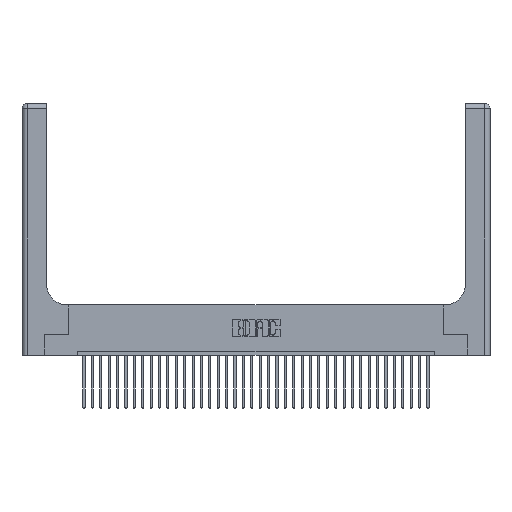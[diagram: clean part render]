
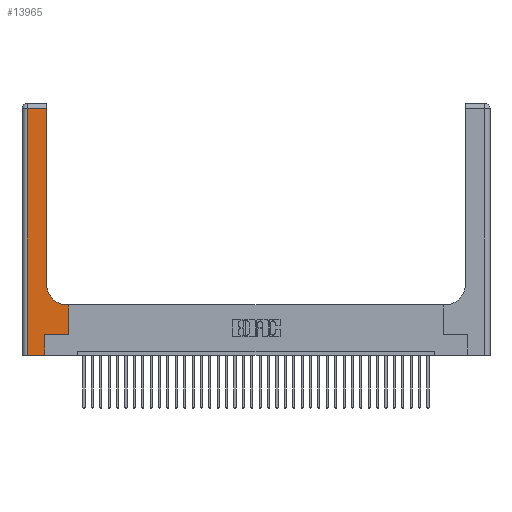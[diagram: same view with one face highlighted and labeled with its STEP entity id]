
A CAD part, top view. The second image highlights one B-rep face of the part: STEP entity #13965.
In plain terms, the highlighted planar face has unit normal (0, 0, 1).
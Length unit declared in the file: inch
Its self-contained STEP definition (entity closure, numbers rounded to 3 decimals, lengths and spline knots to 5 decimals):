
#186 = CARTESIAN_POINT ( 'NONE',  ( 0.269, 0.25, 0.37 ) ) ;
#272 = VERTEX_POINT ( 'NONE', #25800 ) ;
#305 = DIRECTION ( 'NONE',  ( 1., 0., 0. ) ) ;
#426 = VERTEX_POINT ( 'NONE', #12101 ) ;
#628 = CARTESIAN_POINT ( 'NONE',  ( 0.2915, 2.94, 0.37 ) ) ;
#1583 = EDGE_CURVE ( 'NONE', #35221, #21015, #30630, .T. ) ;
#3224 = LINE ( 'NONE', #28354, #12573 ) ;
#3640 = CARTESIAN_POINT ( 'NONE',  ( 0.2915, 3., 0.37 ) ) ;
#4027 = VECTOR ( 'NONE', #305, 39.37008 ) ;
#5336 = LINE ( 'NONE', #30257, #18735 ) ;
#5441 = CARTESIAN_POINT ( 'NONE',  ( 0., 2.94, 0.37 ) ) ;
#5463 = AXIS2_PLACEMENT_3D ( 'NONE', #10043, #32702, #27140 ) ;
#5519 = DIRECTION ( 'NONE',  ( 0., 1., 0. ) ) ;
#6329 = FACE_OUTER_BOUND ( 'NONE', #7974, .T. ) ;
#6881 = EDGE_CURVE ( 'NONE', #22739, #14879, #33818, .T. ) ;
#7729 = ORIENTED_EDGE ( 'NONE', *, *, #27890, .T. ) ;
#7974 = EDGE_LOOP ( 'NONE', ( #9157, #15143, #18791, #7729, #33402, #23126, #13127, #27783, #35935 ) ) ;
#8047 = EDGE_CURVE ( 'NONE', #32085, #272, #3224, .T. ) ;
#8818 = CIRCLE ( 'NONE', #5463, 0.25 ) ;
#9157 = ORIENTED_EDGE ( 'NONE', *, *, #9192, .T. ) ;
#9192 = EDGE_CURVE ( 'NONE', #16877, #10429, #30338, .T. ) ;
#9507 = LINE ( 'NONE', #5441, #30499 ) ;
#9857 = CARTESIAN_POINT ( 'NONE',  ( 0.06, 3., 0.37 ) ) ;
#10043 = CARTESIAN_POINT ( 'NONE',  ( 0.5415, 0.85, 0.37 ) ) ;
#10194 = DIRECTION ( 'NONE',  ( 0., 1., 0. ) ) ;
#10290 = EDGE_CURVE ( 'NONE', #426, #16877, #8818, .T. ) ;
#10429 = VERTEX_POINT ( 'NONE', #628 ) ;
#11141 = DIRECTION ( 'NONE',  ( -1., 0., 0. ) ) ;
#11426 = DIRECTION ( 'NONE',  ( -1., 0., 0. ) ) ;
#12101 = CARTESIAN_POINT ( 'NONE',  ( 0.5415, 0.6, 0.37 ) ) ;
#12436 = VECTOR ( 'NONE', #11141, 39.37008 ) ;
#12573 = VECTOR ( 'NONE', #14466, 39.37008 ) ;
#13127 = ORIENTED_EDGE ( 'NONE', *, *, #6881, .T. ) ;
#13965 = ADVANCED_FACE ( 'NONE', ( #6329 ), #21162, .F. ) ;
#14466 = DIRECTION ( 'NONE',  ( 0., 1., 0. ) ) ;
#14879 = VERTEX_POINT ( 'NONE', #22678 ) ;
#14973 = VECTOR ( 'NONE', #32882, 39.37008 ) ;
#15143 = ORIENTED_EDGE ( 'NONE', *, *, #33697, .T. ) ;
#15558 = VECTOR ( 'NONE', #10194, 39.37008 ) ;
#16877 = VERTEX_POINT ( 'NONE', #29833 ) ;
#16962 = LINE ( 'NONE', #186, #4027 ) ;
#17115 = CARTESIAN_POINT ( 'NONE',  ( 0.5585, 0.25, 0.37 ) ) ;
#18539 = EDGE_CURVE ( 'NONE', #272, #22739, #16962, .T. ) ;
#18735 = VECTOR ( 'NONE', #22133, 39.37008 ) ;
#18791 = ORIENTED_EDGE ( 'NONE', *, *, #1583, .T. ) ;
#21015 = VERTEX_POINT ( 'NONE', #27204 ) ;
#21162 = PLANE ( 'NONE',  #21814 ) ;
#21814 = AXIS2_PLACEMENT_3D ( 'NONE', #35933, #30516, #28621 ) ;
#21847 = CARTESIAN_POINT ( 'NONE',  ( 0.5585, 0.25, 0.37 ) ) ;
#22133 = DIRECTION ( 'NONE',  ( 1., 0., 0. ) ) ;
#22505 = CARTESIAN_POINT ( 'NONE',  ( 0.06, 2.94, 0.37 ) ) ;
#22678 = CARTESIAN_POINT ( 'NONE',  ( 0.5585, 0.6, 0.37 ) ) ;
#22739 = VERTEX_POINT ( 'NONE', #21847 ) ;
#23126 = ORIENTED_EDGE ( 'NONE', *, *, #18539, .T. ) ;
#23465 = EDGE_CURVE ( 'NONE', #14879, #426, #32057, .T. ) ;
#24671 = CARTESIAN_POINT ( 'NONE',  ( 0.269, 0., 0.37 ) ) ;
#25800 = CARTESIAN_POINT ( 'NONE',  ( 0.269, 0.25, 0.37 ) ) ;
#26272 = VECTOR ( 'NONE', #5519, 39.37008 ) ;
#27140 = DIRECTION ( 'NONE',  ( 1., 0., 0. ) ) ;
#27204 = CARTESIAN_POINT ( 'NONE',  ( 0.06, 0., 0.37 ) ) ;
#27783 = ORIENTED_EDGE ( 'NONE', *, *, #23465, .T. ) ;
#27890 = EDGE_CURVE ( 'NONE', #21015, #32085, #5336, .T. ) ;
#28354 = CARTESIAN_POINT ( 'NONE',  ( 0.269, 0., 0.37 ) ) ;
#28621 = DIRECTION ( 'NONE',  ( -1., 0., 0. ) ) ;
#29833 = CARTESIAN_POINT ( 'NONE',  ( 0.2915, 0.85, 0.37 ) ) ;
#30257 = CARTESIAN_POINT ( 'NONE',  ( 0., 0., 0.37 ) ) ;
#30338 = LINE ( 'NONE', #3640, #15558 ) ;
#30499 = VECTOR ( 'NONE', #11426, 39.37008 ) ;
#30516 = DIRECTION ( 'NONE',  ( 0., 0., -1. ) ) ;
#30630 = LINE ( 'NONE', #9857, #14973 ) ;
#30727 = CARTESIAN_POINT ( 'NONE',  ( 0.2915, 0.6, 0.37 ) ) ;
#32057 = LINE ( 'NONE', #30727, #12436 ) ;
#32085 = VERTEX_POINT ( 'NONE', #24671 ) ;
#32702 = DIRECTION ( 'NONE',  ( 0., 0., -1. ) ) ;
#32882 = DIRECTION ( 'NONE',  ( 0., -1., 0. ) ) ;
#33402 = ORIENTED_EDGE ( 'NONE', *, *, #8047, .T. ) ;
#33697 = EDGE_CURVE ( 'NONE', #10429, #35221, #9507, .T. ) ;
#33818 = LINE ( 'NONE', #17115, #26272 ) ;
#35221 = VERTEX_POINT ( 'NONE', #22505 ) ;
#35933 = CARTESIAN_POINT ( 'NONE',  ( 0., 3., 0.37 ) ) ;
#35935 = ORIENTED_EDGE ( 'NONE', *, *, #10290, .T. ) ;
